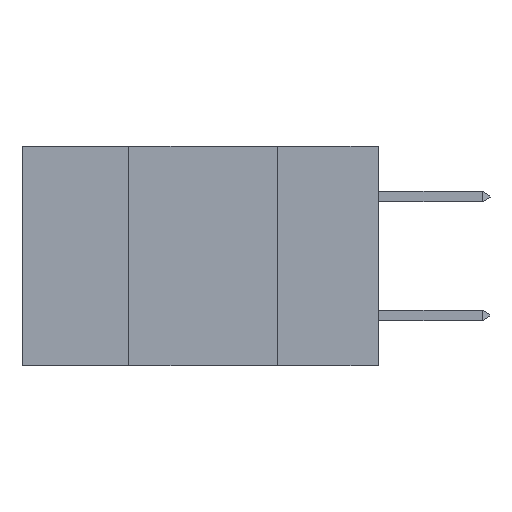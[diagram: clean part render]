
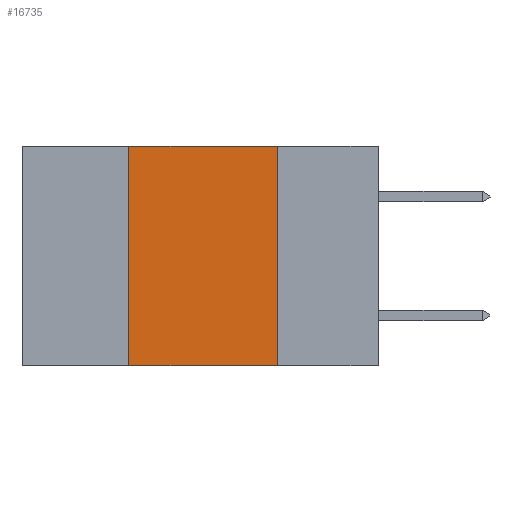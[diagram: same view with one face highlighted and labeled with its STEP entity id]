
A CAD part, left-side view. The second image highlights one B-rep face of the part: STEP entity #16735.
In plain terms, the highlighted planar face has unit normal (-1, 0, 0).
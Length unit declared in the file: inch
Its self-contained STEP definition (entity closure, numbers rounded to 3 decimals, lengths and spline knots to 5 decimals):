
#942 = DIRECTION ( 'NONE',  ( 0., 0., -1. ) ) ;
#1878 = VERTEX_POINT ( 'NONE', #19726 ) ;
#2074 = FACE_OUTER_BOUND ( 'NONE', #24470, .T. ) ;
#3120 = CARTESIAN_POINT ( 'NONE',  ( 0., 0.17, -0.37 ) ) ;
#4679 = ORIENTED_EDGE ( 'NONE', *, *, #6407, .F. ) ;
#5548 = LINE ( 'NONE', #20948, #21072 ) ;
#5987 = ORIENTED_EDGE ( 'NONE', *, *, #25349, .T. ) ;
#6407 = EDGE_CURVE ( 'NONE', #19493, #1878, #25105, .T. ) ;
#6524 = VECTOR ( 'NONE', #942, 39.37008 ) ;
#7197 = DIRECTION ( 'NONE',  ( 0., 0., 1. ) ) ;
#9593 = CARTESIAN_POINT ( 'NONE',  ( 0., 0.6, 0. ) ) ;
#9629 = VERTEX_POINT ( 'NONE', #13725 ) ;
#11735 = DIRECTION ( 'NONE',  ( 0., 0., -1. ) ) ;
#12925 = AXIS2_PLACEMENT_3D ( 'NONE', #9593, #24323, #11735 ) ;
#13084 = CARTESIAN_POINT ( 'NONE',  ( 0., 0.17, -0.37 ) ) ;
#13725 = CARTESIAN_POINT ( 'NONE',  ( 0., 0.42, -0.37 ) ) ;
#14879 = VECTOR ( 'NONE', #7197, 39.37008 ) ;
#15211 = VERTEX_POINT ( 'NONE', #13084 ) ;
#15436 = EDGE_CURVE ( 'NONE', #1878, #15211, #23339, .T. ) ;
#15588 = CARTESIAN_POINT ( 'NONE',  ( 0., 0.42, -0.37 ) ) ;
#16691 = DIRECTION ( 'NONE',  ( 0., -1., 0. ) ) ;
#16735 = ADVANCED_FACE ( 'NONE', ( #2074 ), #17971, .F. ) ;
#17971 = PLANE ( 'NONE',  #12925 ) ;
#19493 = VERTEX_POINT ( 'NONE', #26134 ) ;
#19726 = CARTESIAN_POINT ( 'NONE',  ( 0., 0.17, 0. ) ) ;
#20041 = EDGE_CURVE ( 'NONE', #9629, #19493, #20503, .T. ) ;
#20503 = LINE ( 'NONE', #15588, #14879 ) ;
#20858 = ORIENTED_EDGE ( 'NONE', *, *, #15436, .F. ) ;
#20948 = CARTESIAN_POINT ( 'NONE',  ( 0., 0.6, -0.37 ) ) ;
#21072 = VECTOR ( 'NONE', #16691, 39.37008 ) ;
#22175 = ORIENTED_EDGE ( 'NONE', *, *, #20041, .F. ) ;
#23339 = LINE ( 'NONE', #3120, #6524 ) ;
#23662 = CARTESIAN_POINT ( 'NONE',  ( 0., 0.6, 0. ) ) ;
#24323 = DIRECTION ( 'NONE',  ( 1., 0., 0. ) ) ;
#24470 = EDGE_LOOP ( 'NONE', ( #20858, #4679, #22175, #5987 ) ) ;
#24490 = VECTOR ( 'NONE', #25733, 39.37008 ) ;
#25105 = LINE ( 'NONE', #23662, #24490 ) ;
#25349 = EDGE_CURVE ( 'NONE', #9629, #15211, #5548, .T. ) ;
#25733 = DIRECTION ( 'NONE',  ( 0., -1., 0. ) ) ;
#26134 = CARTESIAN_POINT ( 'NONE',  ( 0., 0.42, 0. ) ) ;
